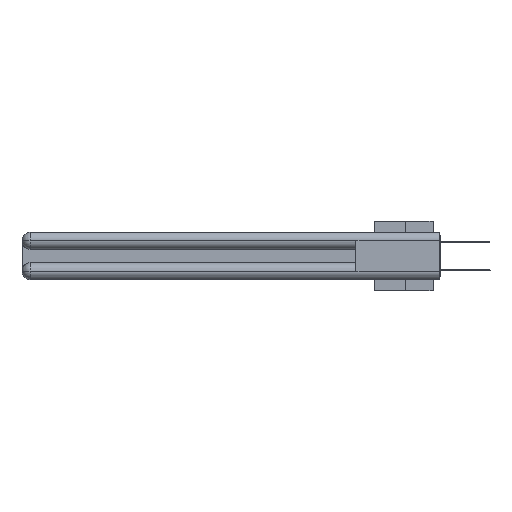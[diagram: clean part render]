
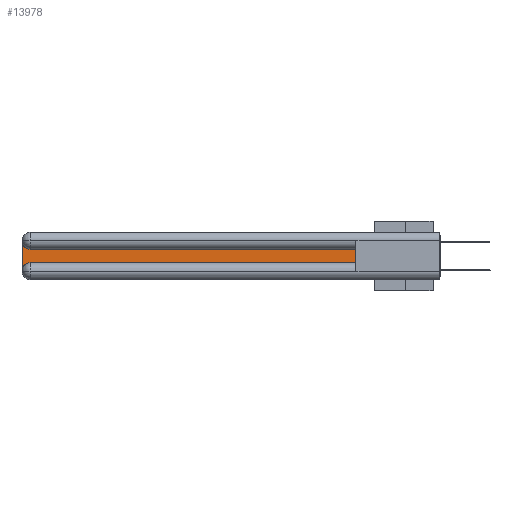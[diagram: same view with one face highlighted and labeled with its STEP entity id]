
A CAD part, left-side view. The second image highlights one B-rep face of the part: STEP entity #13978.
In plain terms, the highlighted planar face has unit normal (-1, 0, 0).
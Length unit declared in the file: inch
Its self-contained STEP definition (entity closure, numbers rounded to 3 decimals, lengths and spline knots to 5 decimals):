
#548 = DIRECTION ( 'NONE',  ( 0., 0., -1. ) ) ;
#1300 = VECTOR ( 'NONE', #4333, 39.37008 ) ;
#1316 = ORIENTED_EDGE ( 'NONE', *, *, #2187, .T. ) ;
#1597 = FACE_OUTER_BOUND ( 'NONE', #3843, .T. ) ;
#2187 = EDGE_CURVE ( 'NONE', #14128, #32575, #13932, .T. ) ;
#2556 = ORIENTED_EDGE ( 'NONE', *, *, #29163, .T. ) ;
#3082 = CIRCLE ( 'NONE', #9702, 0.06 ) ;
#3242 = CARTESIAN_POINT ( 'NONE',  ( 0.075, 2.94, -0.0625 ) ) ;
#3677 = EDGE_CURVE ( 'NONE', #17233, #14128, #9220, .T. ) ;
#3843 = EDGE_LOOP ( 'NONE', ( #27971, #2556, #4754, #1316, #15645, #10310 ) ) ;
#4333 = DIRECTION ( 'NONE',  ( 0., 0., -1. ) ) ;
#4754 = ORIENTED_EDGE ( 'NONE', *, *, #3677, .T. ) ;
#4832 = CARTESIAN_POINT ( 'NONE',  ( 0.075, 3., -0.1225 ) ) ;
#6307 = DIRECTION ( 'NONE',  ( 1., 0., 0. ) ) ;
#6755 = CARTESIAN_POINT ( 'NONE',  ( 0.075, 3., -0.2175 ) ) ;
#7018 = AXIS2_PLACEMENT_3D ( 'NONE', #4832, #10316, #13549 ) ;
#9220 = LINE ( 'NONE', #6755, #1300 ) ;
#9702 = AXIS2_PLACEMENT_3D ( 'NONE', #3242, #18788, #548 ) ;
#10310 = ORIENTED_EDGE ( 'NONE', *, *, #23778, .T. ) ;
#10316 = DIRECTION ( 'NONE',  ( 1., 0., 0. ) ) ;
#11077 = CARTESIAN_POINT ( 'NONE',  ( 0.075, 0.6, -0.2175 ) ) ;
#12488 = VERTEX_POINT ( 'NONE', #11077 ) ;
#13549 = DIRECTION ( 'NONE',  ( 0., 0., -1. ) ) ;
#13932 = CIRCLE ( 'NONE', #22572, 0.06 ) ;
#13978 = ADVANCED_FACE ( 'NONE', ( #1597 ), #18141, .F. ) ;
#14128 = VERTEX_POINT ( 'NONE', #22656 ) ;
#14177 = DIRECTION ( 'NONE',  ( 0., 0., 1. ) ) ;
#14288 = VECTOR ( 'NONE', #19511, 39.37008 ) ;
#14454 = VERTEX_POINT ( 'NONE', #34112 ) ;
#15645 = ORIENTED_EDGE ( 'NONE', *, *, #18722, .T. ) ;
#16939 = CARTESIAN_POINT ( 'NONE',  ( 0.075, 0.6, -0.1225 ) ) ;
#17200 = LINE ( 'NONE', #16939, #14288 ) ;
#17233 = VERTEX_POINT ( 'NONE', #24904 ) ;
#18141 = PLANE ( 'NONE',  #7018 ) ;
#18722 = EDGE_CURVE ( 'NONE', #32575, #12488, #23165, .T. ) ;
#18788 = DIRECTION ( 'NONE',  ( 1., 0., 0. ) ) ;
#18799 = LINE ( 'NONE', #32990, #22125 ) ;
#19511 = DIRECTION ( 'NONE',  ( 0., 1., 0. ) ) ;
#20224 = VECTOR ( 'NONE', #24676, 39.37008 ) ;
#21143 = CARTESIAN_POINT ( 'NONE',  ( 0.075, 2.94, -0.2775 ) ) ;
#21245 = VERTEX_POINT ( 'NONE', #23291 ) ;
#22125 = VECTOR ( 'NONE', #14177, 39.37008 ) ;
#22401 = EDGE_CURVE ( 'NONE', #21245, #14454, #17200, .T. ) ;
#22572 = AXIS2_PLACEMENT_3D ( 'NONE', #21143, #6307, #23724 ) ;
#22656 = CARTESIAN_POINT ( 'NONE',  ( 0.075, 3., -0.2775 ) ) ;
#23165 = LINE ( 'NONE', #29496, #20224 ) ;
#23291 = CARTESIAN_POINT ( 'NONE',  ( 0.075, 0.6, -0.1225 ) ) ;
#23724 = DIRECTION ( 'NONE',  ( 0., 0., -1. ) ) ;
#23778 = EDGE_CURVE ( 'NONE', #12488, #21245, #18799, .T. ) ;
#24676 = DIRECTION ( 'NONE',  ( 0., -1., 0. ) ) ;
#24904 = CARTESIAN_POINT ( 'NONE',  ( 0.075, 3., -0.0625 ) ) ;
#25177 = CARTESIAN_POINT ( 'NONE',  ( 0.075, 2.94, -0.2175 ) ) ;
#27971 = ORIENTED_EDGE ( 'NONE', *, *, #22401, .T. ) ;
#29163 = EDGE_CURVE ( 'NONE', #14454, #17233, #3082, .T. ) ;
#29496 = CARTESIAN_POINT ( 'NONE',  ( 0.075, 0.6, -0.2175 ) ) ;
#32575 = VERTEX_POINT ( 'NONE', #25177 ) ;
#32990 = CARTESIAN_POINT ( 'NONE',  ( 0.075, 0.6, -0.2175 ) ) ;
#34112 = CARTESIAN_POINT ( 'NONE',  ( 0.075, 2.94, -0.1225 ) ) ;
